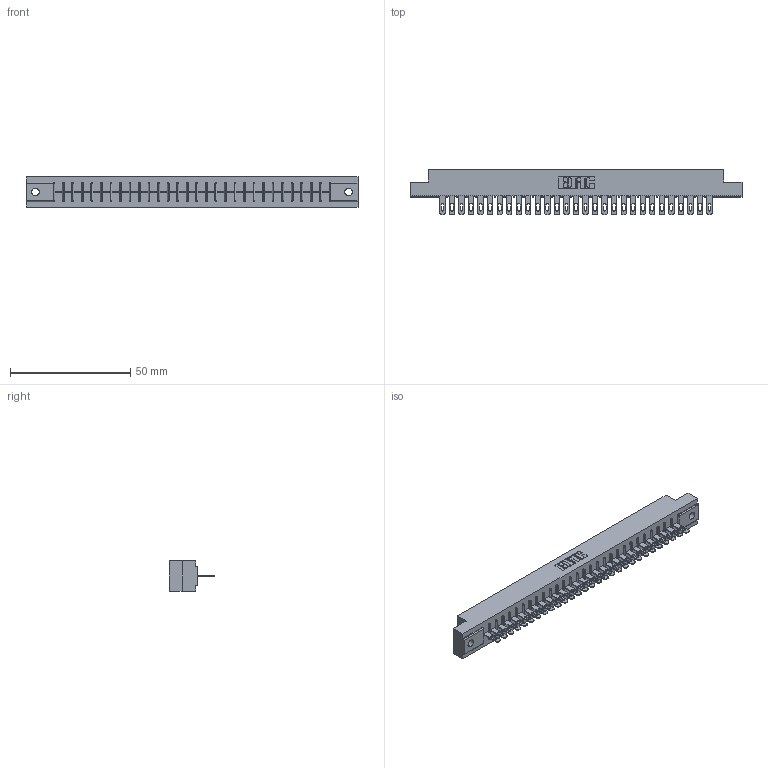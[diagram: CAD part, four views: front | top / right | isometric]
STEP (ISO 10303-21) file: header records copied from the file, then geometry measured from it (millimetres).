
FILE_DESCRIPTION (( 'STEP AP203' ), '1' );
FILE_NAME ('316-029-400-102.STEP', '2020-09-22T23:46:31', ( '' ), ( '' ), 'SwSTEP 2.0', 'SolidWorks 2020', '' );
FILE_SCHEMA (( 'CONFIG_CONTROL_DESIGN' ));
Length unit declared in the file: inch
Products named in the file (3): 306 Part_.128 Dia; 316-029-400-102; 306-290-001_100
Assembly tree (30 placements, depth 2):
  316-029-400-102
    306 Part_.128 Dia
    306-290-001_100  x29
Bounding box: 137.92 x 18.87 x 12.7 mm (x, y, z)
Volume: 15195.4 mm3; surface area: 15679.8 mm2
Topology: 30 solids, 30 shells, 2320 faces, 6551 edges, 4210 vertices
Faces by surface type: plane 1518, cylinder 686, sphere 116
Entity records: 28894 total; most frequent: CARTESIAN_POINT 4850, ORIENTED_EDGE 4806, DIRECTION 4785, EDGE_CURVE 2403, LINE 1871, VECTOR 1871, VERTEX_POINT 1522, AXIS2_PLACEMENT_3D 1457
